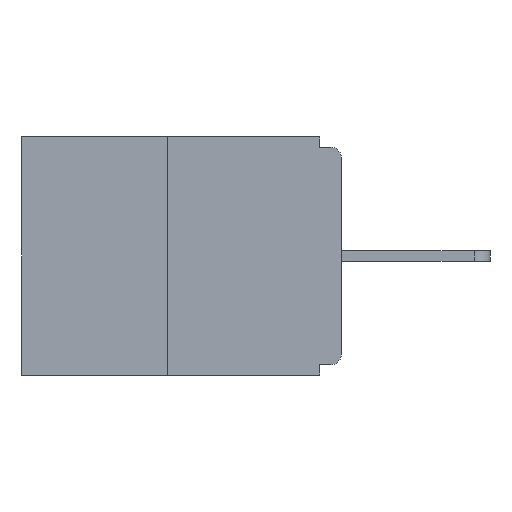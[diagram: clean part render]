
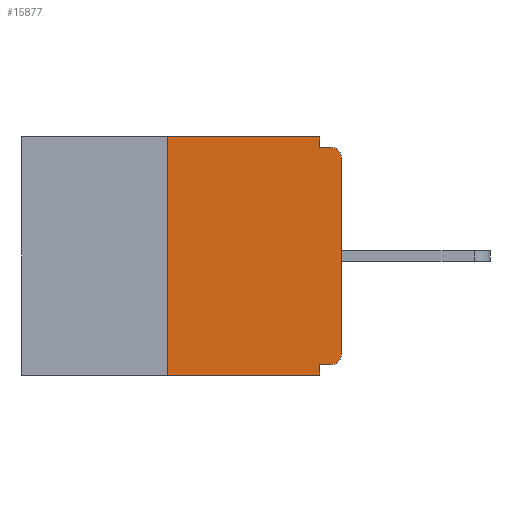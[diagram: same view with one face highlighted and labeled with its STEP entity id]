
A CAD part, left-side view. The second image highlights one B-rep face of the part: STEP entity #15877.
In plain terms, the highlighted planar face has unit normal (-1, 0, 0).
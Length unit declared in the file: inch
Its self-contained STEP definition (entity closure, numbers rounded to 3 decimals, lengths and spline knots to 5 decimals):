
#495 = DIRECTION ( 'NONE',  ( 0., 0., 1. ) ) ;
#656 = CARTESIAN_POINT ( 'NONE',  ( 0., 0., -0.328 ) ) ;
#780 = DIRECTION ( 'NONE',  ( 0., 1., 0. ) ) ;
#785 = CIRCLE ( 'NONE', #1739, 0.015 ) ;
#1739 = AXIS2_PLACEMENT_3D ( 'NONE', #15474, #6993, #16825 ) ;
#1850 = CARTESIAN_POINT ( 'NONE',  ( 0., 0.031, 0. ) ) ;
#1990 = CARTESIAN_POINT ( 'NONE',  ( 0., 0., -0.03 ) ) ;
#2004 = LINE ( 'NONE', #6457, #16791 ) ;
#2039 = ORIENTED_EDGE ( 'NONE', *, *, #9843, .F. ) ;
#2404 = CARTESIAN_POINT ( 'NONE',  ( 0., 0., -0.313 ) ) ;
#2521 = LINE ( 'NONE', #5605, #17244 ) ;
#2895 = CARTESIAN_POINT ( 'NONE',  ( 0., 0.46, 0. ) ) ;
#3125 = VERTEX_POINT ( 'NONE', #17083 ) ;
#3661 = CARTESIAN_POINT ( 'NONE',  ( 0., 0.46, -0.343 ) ) ;
#3799 = AXIS2_PLACEMENT_3D ( 'NONE', #14963, #6437, #16301 ) ;
#3869 = CARTESIAN_POINT ( 'NONE',  ( 0., 0.031, 0. ) ) ;
#4154 = VERTEX_POINT ( 'NONE', #7197 ) ;
#4211 = VERTEX_POINT ( 'NONE', #8071 ) ;
#4620 = ORIENTED_EDGE ( 'NONE', *, *, #10156, .F. ) ;
#4715 = DIRECTION ( 'NONE',  ( 0., -1., 0. ) ) ;
#5092 = ORIENTED_EDGE ( 'NONE', *, *, #5939, .F. ) ;
#5424 = DIRECTION ( 'NONE',  ( 0., 0., 1. ) ) ;
#5460 = EDGE_CURVE ( 'NONE', #3125, #17689, #2521, .T. ) ;
#5553 = ORIENTED_EDGE ( 'NONE', *, *, #14562, .T. ) ;
#5605 = CARTESIAN_POINT ( 'NONE',  ( 0., 0.25, 0. ) ) ;
#5769 = DIRECTION ( 'NONE',  ( 0., 0., -1. ) ) ;
#5905 = PLANE ( 'NONE',  #11840 ) ;
#5939 = EDGE_CURVE ( 'NONE', #12095, #4211, #2004, .T. ) ;
#6018 = ORIENTED_EDGE ( 'NONE', *, *, #8594, .F. ) ;
#6076 = LINE ( 'NONE', #17380, #17312 ) ;
#6364 = DIRECTION ( 'NONE',  ( 0., 0., -1. ) ) ;
#6368 = VECTOR ( 'NONE', #6364, 39.37008 ) ;
#6437 = DIRECTION ( 'NONE',  ( -1., 0., 0. ) ) ;
#6457 = CARTESIAN_POINT ( 'NONE',  ( 0., 0.031, -0.343 ) ) ;
#6467 = EDGE_LOOP ( 'NONE', ( #4620, #8501, #12415, #5092, #8964, #12838, #5553, #9442, #2039, #6018 ) ) ;
#6993 = DIRECTION ( 'NONE',  ( -1., 0., 0. ) ) ;
#7033 = CIRCLE ( 'NONE', #3799, 0.015 ) ;
#7094 = EDGE_CURVE ( 'NONE', #18026, #12095, #13829, .T. ) ;
#7197 = CARTESIAN_POINT ( 'NONE',  ( 0., 0.031, -0.015 ) ) ;
#7347 = DIRECTION ( 'NONE',  ( 0., 0., -1. ) ) ;
#8071 = CARTESIAN_POINT ( 'NONE',  ( 0., 0.031, -0.343 ) ) ;
#8361 = CARTESIAN_POINT ( 'NONE',  ( 0., 0.015, -0.015 ) ) ;
#8501 = ORIENTED_EDGE ( 'NONE', *, *, #5460, .F. ) ;
#8594 = EDGE_CURVE ( 'NONE', #17933, #4154, #10232, .T. ) ;
#8964 = ORIENTED_EDGE ( 'NONE', *, *, #7094, .F. ) ;
#9055 = CARTESIAN_POINT ( 'NONE',  ( 0., 0., -0.015 ) ) ;
#9236 = FACE_OUTER_BOUND ( 'NONE', #6467, .T. ) ;
#9355 = CARTESIAN_POINT ( 'NONE',  ( 0., 0.031, -0.328 ) ) ;
#9442 = ORIENTED_EDGE ( 'NONE', *, *, #14511, .T. ) ;
#9541 = VECTOR ( 'NONE', #495, 39.37008 ) ;
#9843 = EDGE_CURVE ( 'NONE', #4154, #11157, #11616, .T. ) ;
#9960 = CARTESIAN_POINT ( 'NONE',  ( 0., 0.015, -0.328 ) ) ;
#10156 = EDGE_CURVE ( 'NONE', #17689, #17933, #6076, .T. ) ;
#10232 = LINE ( 'NONE', #1850, #6368 ) ;
#10502 = DIRECTION ( 'NONE',  ( 0., -1., 0. ) ) ;
#11157 = VERTEX_POINT ( 'NONE', #8361 ) ;
#11263 = VECTOR ( 'NONE', #12526, 39.37008 ) ;
#11616 = LINE ( 'NONE', #9055, #18405 ) ;
#11840 = AXIS2_PLACEMENT_3D ( 'NONE', #2895, #15814, #7347 ) ;
#12095 = VERTEX_POINT ( 'NONE', #9355 ) ;
#12104 = VERTEX_POINT ( 'NONE', #1990 ) ;
#12303 = EDGE_CURVE ( 'NONE', #18026, #17342, #785, .T. ) ;
#12415 = ORIENTED_EDGE ( 'NONE', *, *, #12757, .T. ) ;
#12526 = DIRECTION ( 'NONE',  ( 0., -1., 0. ) ) ;
#12757 = EDGE_CURVE ( 'NONE', #3125, #4211, #18506, .T. ) ;
#12838 = ORIENTED_EDGE ( 'NONE', *, *, #12303, .T. ) ;
#13354 = LINE ( 'NONE', #13684, #9541 ) ;
#13419 = CARTESIAN_POINT ( 'NONE',  ( 0., 0.25, 0. ) ) ;
#13684 = CARTESIAN_POINT ( 'NONE',  ( 0., 0., 0. ) ) ;
#13829 = LINE ( 'NONE', #656, #16535 ) ;
#14511 = EDGE_CURVE ( 'NONE', #12104, #11157, #7033, .T. ) ;
#14562 = EDGE_CURVE ( 'NONE', #17342, #12104, #13354, .T. ) ;
#14963 = CARTESIAN_POINT ( 'NONE',  ( 0., 0.015, -0.03 ) ) ;
#15474 = CARTESIAN_POINT ( 'NONE',  ( 0., 0.015, -0.313 ) ) ;
#15814 = DIRECTION ( 'NONE',  ( 1., 0., 0. ) ) ;
#15877 = ADVANCED_FACE ( 'NONE', ( #9236 ), #5905, .F. ) ;
#16301 = DIRECTION ( 'NONE',  ( 0., 0., -1. ) ) ;
#16535 = VECTOR ( 'NONE', #780, 39.37008 ) ;
#16791 = VECTOR ( 'NONE', #5769, 39.37008 ) ;
#16825 = DIRECTION ( 'NONE',  ( 0., 0., -1. ) ) ;
#17083 = CARTESIAN_POINT ( 'NONE',  ( 0., 0.25, -0.343 ) ) ;
#17244 = VECTOR ( 'NONE', #5424, 39.37008 ) ;
#17312 = VECTOR ( 'NONE', #10502, 39.37008 ) ;
#17342 = VERTEX_POINT ( 'NONE', #2404 ) ;
#17380 = CARTESIAN_POINT ( 'NONE',  ( 0., 0.46, 0. ) ) ;
#17689 = VERTEX_POINT ( 'NONE', #13419 ) ;
#17933 = VERTEX_POINT ( 'NONE', #3869 ) ;
#18026 = VERTEX_POINT ( 'NONE', #9960 ) ;
#18405 = VECTOR ( 'NONE', #4715, 39.37008 ) ;
#18506 = LINE ( 'NONE', #3661, #11263 ) ;
